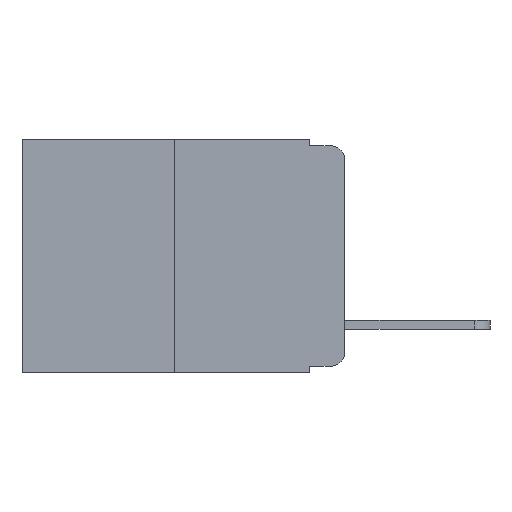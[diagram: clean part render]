
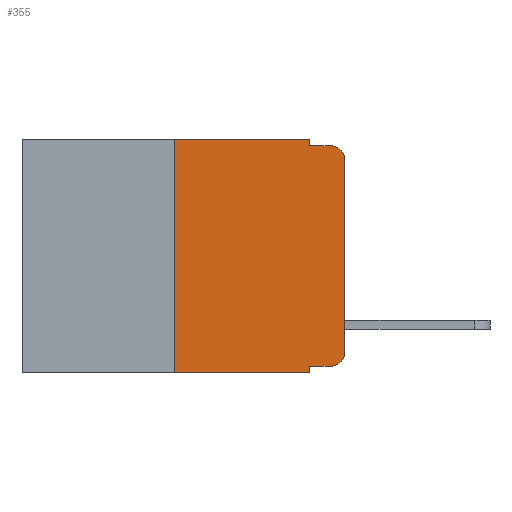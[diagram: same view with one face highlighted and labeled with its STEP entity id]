
A CAD part, left-side view. The second image highlights one B-rep face of the part: STEP entity #355.
In plain terms, the highlighted planar face has unit normal (-1, 0, 0).
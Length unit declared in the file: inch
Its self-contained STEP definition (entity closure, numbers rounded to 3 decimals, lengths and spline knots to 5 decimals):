
#141 = CARTESIAN_POINT ( 'NONE',  ( 0., 0., -0.03 ) ) ;
#152 = LINE ( 'NONE', #12621, #3076 ) ;
#355 = ADVANCED_FACE ( 'NONE', ( #4965 ), #4059, .F. ) ;
#550 = CIRCLE ( 'NONE', #1606, 0.02 ) ;
#800 = CARTESIAN_POINT ( 'NONE',  ( 0., 0.051, -0.343 ) ) ;
#889 = CARTESIAN_POINT ( 'NONE',  ( 0., 0.25, 0. ) ) ;
#965 = CIRCLE ( 'NONE', #7312, 0.02 ) ;
#1179 = CARTESIAN_POINT ( 'NONE',  ( 0., 0.02, -0.313 ) ) ;
#1606 = AXIS2_PLACEMENT_3D ( 'NONE', #8801, #2500, #9816 ) ;
#2189 = VERTEX_POINT ( 'NONE', #141 ) ;
#2206 = DIRECTION ( 'NONE',  ( 0., 0., -1. ) ) ;
#2450 = DIRECTION ( 'NONE',  ( 0., 0., 1. ) ) ;
#2462 = DIRECTION ( 'NONE',  ( 0., 0., -1. ) ) ;
#2500 = DIRECTION ( 'NONE',  ( -1., 0., 0. ) ) ;
#2553 = VECTOR ( 'NONE', #10476, 39.37008 ) ;
#2563 = ORIENTED_EDGE ( 'NONE', *, *, #4502, .T. ) ;
#2841 = VERTEX_POINT ( 'NONE', #3711 ) ;
#2886 = ORIENTED_EDGE ( 'NONE', *, *, #8751, .T. ) ;
#3076 = VECTOR ( 'NONE', #6800, 39.37008 ) ;
#3081 = CARTESIAN_POINT ( 'NONE',  ( 0., 0.051, 0. ) ) ;
#3084 = ORIENTED_EDGE ( 'NONE', *, *, #9194, .T. ) ;
#3314 = CARTESIAN_POINT ( 'NONE',  ( 0., 0.051, 0. ) ) ;
#3560 = CARTESIAN_POINT ( 'NONE',  ( 0., 0., -0.313 ) ) ;
#3711 = CARTESIAN_POINT ( 'NONE',  ( 0., 0.02, -0.333 ) ) ;
#3859 = VERTEX_POINT ( 'NONE', #5101 ) ;
#4059 = PLANE ( 'NONE',  #8814 ) ;
#4068 = VECTOR ( 'NONE', #2450, 39.37008 ) ;
#4073 = CARTESIAN_POINT ( 'NONE',  ( 0., 0.473, 0. ) ) ;
#4206 = ORIENTED_EDGE ( 'NONE', *, *, #9015, .F. ) ;
#4283 = DIRECTION ( 'NONE',  ( 0., 0., -1. ) ) ;
#4502 = EDGE_CURVE ( 'NONE', #3859, #7249, #11647, .T. ) ;
#4549 = DIRECTION ( 'NONE',  ( 1., 0., 0. ) ) ;
#4785 = EDGE_LOOP ( 'NONE', ( #10182, #2886, #13463, #4206, #7990, #12060, #2563, #6052, #6388, #3084 ) ) ;
#4853 = DIRECTION ( 'NONE',  ( 0., -1., 0. ) ) ;
#4964 = CARTESIAN_POINT ( 'NONE',  ( 0., 0.051, -0.333 ) ) ;
#4965 = FACE_OUTER_BOUND ( 'NONE', #4785, .T. ) ;
#5033 = CARTESIAN_POINT ( 'NONE',  ( 0., 0.473, 0. ) ) ;
#5101 = CARTESIAN_POINT ( 'NONE',  ( 0., 0.25, -0.343 ) ) ;
#5166 = LINE ( 'NONE', #4073, #12741 ) ;
#5395 = CARTESIAN_POINT ( 'NONE',  ( 0., 0.25, 0. ) ) ;
#5702 = VECTOR ( 'NONE', #4283, 39.37008 ) ;
#6052 = ORIENTED_EDGE ( 'NONE', *, *, #9074, .F. ) ;
#6159 = VERTEX_POINT ( 'NONE', #889 ) ;
#6316 = VERTEX_POINT ( 'NONE', #6860 ) ;
#6371 = CARTESIAN_POINT ( 'NONE',  ( 0., 0.051, 0. ) ) ;
#6388 = ORIENTED_EDGE ( 'NONE', *, *, #9154, .T. ) ;
#6602 = CARTESIAN_POINT ( 'NONE',  ( 0., 0.051, -0.01 ) ) ;
#6635 = DIRECTION ( 'NONE',  ( 0., -1., 0. ) ) ;
#6800 = DIRECTION ( 'NONE',  ( 0., -1., 0. ) ) ;
#6860 = CARTESIAN_POINT ( 'NONE',  ( 0., 0.02, -0.01 ) ) ;
#7167 = LINE ( 'NONE', #13329, #9602 ) ;
#7249 = VERTEX_POINT ( 'NONE', #800 ) ;
#7312 = AXIS2_PLACEMENT_3D ( 'NONE', #1179, #8766, #2462 ) ;
#7900 = VERTEX_POINT ( 'NONE', #6602 ) ;
#7990 = ORIENTED_EDGE ( 'NONE', *, *, #10269, .F. ) ;
#8005 = VERTEX_POINT ( 'NONE', #3560 ) ;
#8149 = LINE ( 'NONE', #5395, #2553 ) ;
#8331 = VERTEX_POINT ( 'NONE', #4964 ) ;
#8471 = LINE ( 'NONE', #6371, #5702 ) ;
#8499 = VERTEX_POINT ( 'NONE', #3081 ) ;
#8734 = EDGE_CURVE ( 'NONE', #8005, #2189, #9296, .T. ) ;
#8751 = EDGE_CURVE ( 'NONE', #2189, #6316, #550, .T. ) ;
#8766 = DIRECTION ( 'NONE',  ( -1., 0., 0. ) ) ;
#8801 = CARTESIAN_POINT ( 'NONE',  ( 0., 0.02, -0.03 ) ) ;
#8810 = EDGE_CURVE ( 'NONE', #7900, #6316, #152, .T. ) ;
#8814 = AXIS2_PLACEMENT_3D ( 'NONE', #5033, #4549, #10376 ) ;
#9015 = EDGE_CURVE ( 'NONE', #8499, #7900, #8471, .T. ) ;
#9056 = EDGE_CURVE ( 'NONE', #3859, #6159, #8149, .T. ) ;
#9074 = EDGE_CURVE ( 'NONE', #8331, #7249, #12907, .T. ) ;
#9154 = EDGE_CURVE ( 'NONE', #8331, #2841, #7167, .T. ) ;
#9194 = EDGE_CURVE ( 'NONE', #2841, #8005, #965, .T. ) ;
#9296 = LINE ( 'NONE', #9775, #4068 ) ;
#9324 = DIRECTION ( 'NONE',  ( 0., -1., 0. ) ) ;
#9602 = VECTOR ( 'NONE', #6635, 39.37008 ) ;
#9775 = CARTESIAN_POINT ( 'NONE',  ( 0., 0., 0. ) ) ;
#9816 = DIRECTION ( 'NONE',  ( 0., 0., -1. ) ) ;
#10182 = ORIENTED_EDGE ( 'NONE', *, *, #8734, .T. ) ;
#10269 = EDGE_CURVE ( 'NONE', #6159, #8499, #5166, .T. ) ;
#10376 = DIRECTION ( 'NONE',  ( 0., 0., -1. ) ) ;
#10476 = DIRECTION ( 'NONE',  ( 0., 0., 1. ) ) ;
#10761 = VECTOR ( 'NONE', #2206, 39.37008 ) ;
#11647 = LINE ( 'NONE', #12820, #12775 ) ;
#12060 = ORIENTED_EDGE ( 'NONE', *, *, #9056, .F. ) ;
#12621 = CARTESIAN_POINT ( 'NONE',  ( 0., 0.051, -0.01 ) ) ;
#12741 = VECTOR ( 'NONE', #9324, 39.37008 ) ;
#12775 = VECTOR ( 'NONE', #4853, 39.37008 ) ;
#12820 = CARTESIAN_POINT ( 'NONE',  ( 0., 0.473, -0.343 ) ) ;
#12907 = LINE ( 'NONE', #3314, #10761 ) ;
#13329 = CARTESIAN_POINT ( 'NONE',  ( 0., 0.051, -0.333 ) ) ;
#13463 = ORIENTED_EDGE ( 'NONE', *, *, #8810, .F. ) ;
